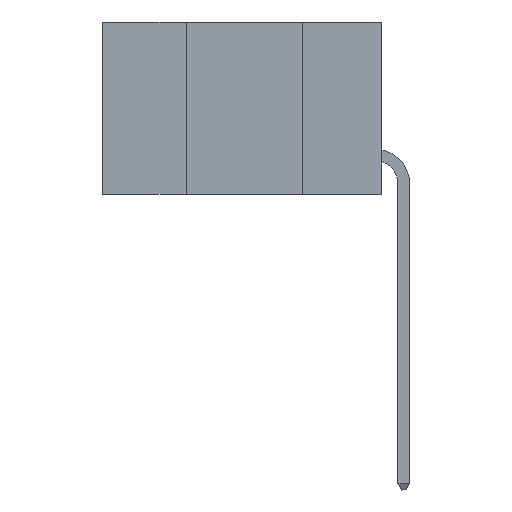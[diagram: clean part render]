
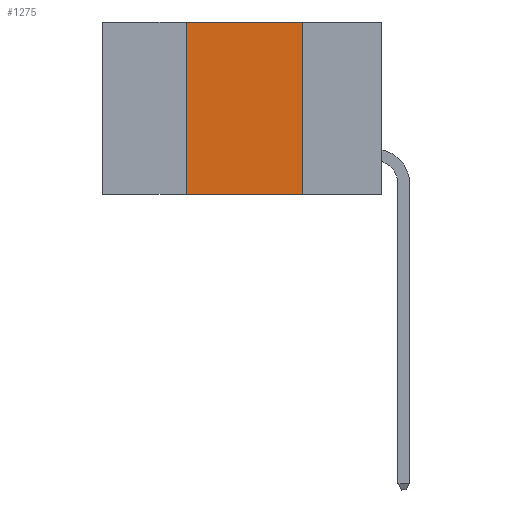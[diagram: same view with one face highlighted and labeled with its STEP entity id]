
A CAD part, left-side view. The second image highlights one B-rep face of the part: STEP entity #1275.
In plain terms, the highlighted planar face has unit normal (-1, 0, 0).
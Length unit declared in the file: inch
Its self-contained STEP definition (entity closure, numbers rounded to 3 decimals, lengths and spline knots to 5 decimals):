
#61 = LINE ( 'NONE', #14676, #6790 ) ;
#312 = CARTESIAN_POINT ( 'NONE',  ( 0., 0.42, 0. ) ) ;
#459 = LINE ( 'NONE', #13987, #7549 ) ;
#499 = CARTESIAN_POINT ( 'NONE',  ( 0., 0.17, 0. ) ) ;
#944 = EDGE_CURVE ( 'NONE', #6426, #12997, #5905, .T. ) ;
#1275 = ADVANCED_FACE ( 'NONE', ( #10538 ), #10816, .F. ) ;
#1551 = ORIENTED_EDGE ( 'NONE', *, *, #12215, .F. ) ;
#1591 = VECTOR ( 'NONE', #10951, 39.37008 ) ;
#1595 = CARTESIAN_POINT ( 'NONE',  ( 0., 0.42, -0.37 ) ) ;
#2332 = VERTEX_POINT ( 'NONE', #9536 ) ;
#2586 = DIRECTION ( 'NONE',  ( 0., 0., 1. ) ) ;
#2612 = EDGE_CURVE ( 'NONE', #9603, #2332, #61, .T. ) ;
#2630 = CARTESIAN_POINT ( 'NONE',  ( 0., 0.6, 0. ) ) ;
#2972 = ORIENTED_EDGE ( 'NONE', *, *, #10380, .F. ) ;
#5905 = LINE ( 'NONE', #14990, #14184 ) ;
#5963 = ORIENTED_EDGE ( 'NONE', *, *, #2612, .F. ) ;
#6103 = DIRECTION ( 'NONE',  ( 1., 0., 0. ) ) ;
#6153 = DIRECTION ( 'NONE',  ( 0., 0., -1. ) ) ;
#6426 = VERTEX_POINT ( 'NONE', #1595 ) ;
#6790 = VECTOR ( 'NONE', #7427, 39.37008 ) ;
#6841 = AXIS2_PLACEMENT_3D ( 'NONE', #2630, #6103, #6153 ) ;
#7427 = DIRECTION ( 'NONE',  ( 0., -1., 0. ) ) ;
#7549 = VECTOR ( 'NONE', #2586, 39.37008 ) ;
#8622 = CARTESIAN_POINT ( 'NONE',  ( 0., 0.17, -0.37 ) ) ;
#9536 = CARTESIAN_POINT ( 'NONE',  ( 0., 0.17, 0. ) ) ;
#9603 = VERTEX_POINT ( 'NONE', #312 ) ;
#10270 = DIRECTION ( 'NONE',  ( 0., -1., 0. ) ) ;
#10380 = EDGE_CURVE ( 'NONE', #6426, #9603, #459, .T. ) ;
#10538 = FACE_OUTER_BOUND ( 'NONE', #10718, .T. ) ;
#10718 = EDGE_LOOP ( 'NONE', ( #1551, #5963, #2972, #11565 ) ) ;
#10816 = PLANE ( 'NONE',  #6841 ) ;
#10951 = DIRECTION ( 'NONE',  ( 0., 0., -1. ) ) ;
#11565 = ORIENTED_EDGE ( 'NONE', *, *, #944, .T. ) ;
#12215 = EDGE_CURVE ( 'NONE', #2332, #12997, #14425, .T. ) ;
#12997 = VERTEX_POINT ( 'NONE', #8622 ) ;
#13987 = CARTESIAN_POINT ( 'NONE',  ( 0., 0.42, 0. ) ) ;
#14184 = VECTOR ( 'NONE', #10270, 39.37008 ) ;
#14425 = LINE ( 'NONE', #499, #1591 ) ;
#14676 = CARTESIAN_POINT ( 'NONE',  ( 0., 0.6, 0. ) ) ;
#14990 = CARTESIAN_POINT ( 'NONE',  ( 0., 0.6, -0.37 ) ) ;
